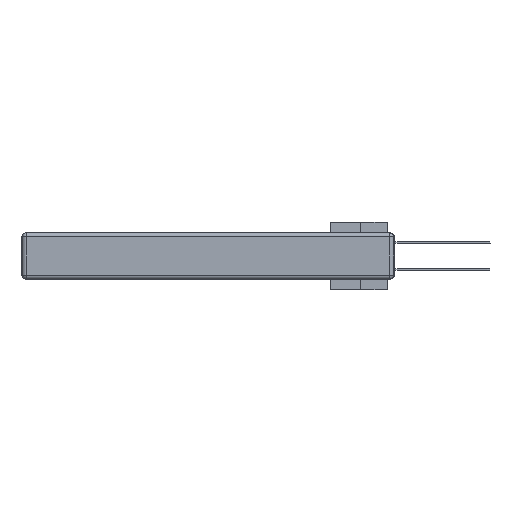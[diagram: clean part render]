
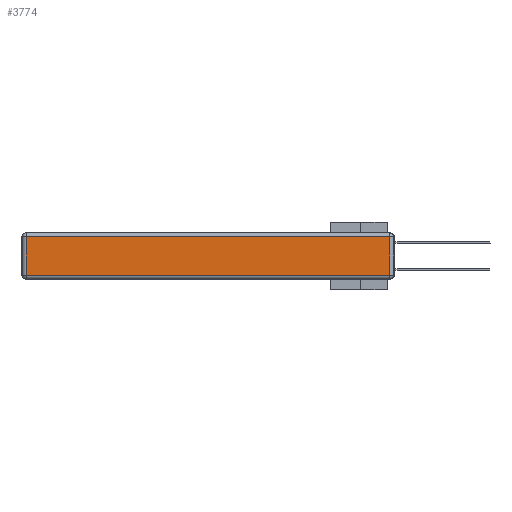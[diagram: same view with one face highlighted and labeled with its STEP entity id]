
A CAD part, left-side view. The second image highlights one B-rep face of the part: STEP entity #3774.
In plain terms, the highlighted planar face has unit normal (-1, 0, 0).
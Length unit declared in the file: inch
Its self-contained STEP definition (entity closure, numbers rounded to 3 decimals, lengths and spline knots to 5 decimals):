
#2181 = ORIENTED_EDGE ( 'NONE', *, *, #23168, .T. ) ;
#3774 = ADVANCED_FACE ( 'NONE', ( #27634 ), #9183, .T. ) ;
#4124 = DIRECTION ( 'NONE',  ( 0., 1., 0. ) ) ;
#6800 = CARTESIAN_POINT ( 'NONE',  ( 0., 2.72, -0.313 ) ) ;
#7005 = DIRECTION ( 'NONE',  ( 0., 0., 1. ) ) ;
#9183 = PLANE ( 'NONE',  #17388 ) ;
#10073 = DIRECTION ( 'NONE',  ( 0., -1., 0. ) ) ;
#10481 = CARTESIAN_POINT ( 'NONE',  ( 0., 0.03, -0.313 ) ) ;
#13348 = LINE ( 'NONE', #31293, #37563 ) ;
#14197 = VECTOR ( 'NONE', #7005, 39.37008 ) ;
#15963 = DIRECTION ( 'NONE',  ( 0., 0., -1. ) ) ;
#16313 = ORIENTED_EDGE ( 'NONE', *, *, #27101, .T. ) ;
#17388 = AXIS2_PLACEMENT_3D ( 'NONE', #30976, #40763, #28741 ) ;
#19278 = CARTESIAN_POINT ( 'NONE',  ( 0., 2.75, -0.03 ) ) ;
#20034 = LINE ( 'NONE', #35867, #33477 ) ;
#21461 = EDGE_CURVE ( 'NONE', #27527, #24402, #23002, .T. ) ;
#22803 = CARTESIAN_POINT ( 'NONE',  ( 0., 0.03, -0.343 ) ) ;
#22963 = CARTESIAN_POINT ( 'NONE',  ( 0., 2.72, -0.03 ) ) ;
#23002 = LINE ( 'NONE', #22803, #14197 ) ;
#23168 = EDGE_CURVE ( 'NONE', #24402, #24997, #39103, .T. ) ;
#23909 = VERTEX_POINT ( 'NONE', #6800 ) ;
#24402 = VERTEX_POINT ( 'NONE', #34298 ) ;
#24997 = VERTEX_POINT ( 'NONE', #22963 ) ;
#25703 = EDGE_LOOP ( 'NONE', ( #16313, #38328, #2181, #33687 ) ) ;
#27101 = EDGE_CURVE ( 'NONE', #23909, #27527, #20034, .T. ) ;
#27527 = VERTEX_POINT ( 'NONE', #10481 ) ;
#27634 = FACE_OUTER_BOUND ( 'NONE', #25703, .T. ) ;
#28741 = DIRECTION ( 'NONE',  ( 0., 0., 1. ) ) ;
#30725 = VECTOR ( 'NONE', #4124, 39.37008 ) ;
#30925 = EDGE_CURVE ( 'NONE', #24997, #23909, #13348, .T. ) ;
#30976 = CARTESIAN_POINT ( 'NONE',  ( 0., 0., -0.343 ) ) ;
#31293 = CARTESIAN_POINT ( 'NONE',  ( 0., 2.72, -0.343 ) ) ;
#33477 = VECTOR ( 'NONE', #10073, 39.37008 ) ;
#33687 = ORIENTED_EDGE ( 'NONE', *, *, #30925, .T. ) ;
#34298 = CARTESIAN_POINT ( 'NONE',  ( 0., 0.03, -0.03 ) ) ;
#35867 = CARTESIAN_POINT ( 'NONE',  ( 0., 0., -0.313 ) ) ;
#37563 = VECTOR ( 'NONE', #15963, 39.37008 ) ;
#38328 = ORIENTED_EDGE ( 'NONE', *, *, #21461, .T. ) ;
#39103 = LINE ( 'NONE', #19278, #30725 ) ;
#40763 = DIRECTION ( 'NONE',  ( -1., 0., 0. ) ) ;
